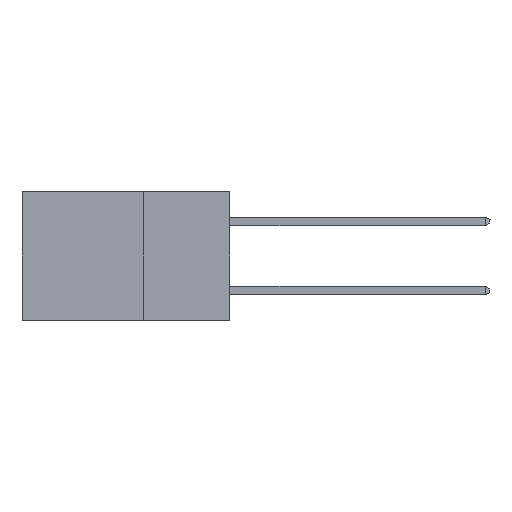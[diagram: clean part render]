
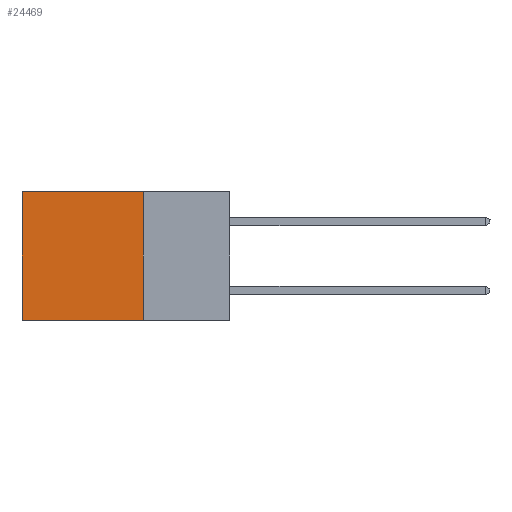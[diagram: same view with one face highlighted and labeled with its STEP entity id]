
A CAD part, left-side view. The second image highlights one B-rep face of the part: STEP entity #24469.
In plain terms, the highlighted planar face has unit normal (-1, 0, 0).
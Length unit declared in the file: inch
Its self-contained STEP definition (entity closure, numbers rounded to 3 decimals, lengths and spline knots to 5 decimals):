
#397 = CARTESIAN_POINT ( 'NONE',  ( 0.298, 0.6, 0. ) ) ;
#548 = FACE_OUTER_BOUND ( 'NONE', #2076, .T. ) ;
#900 = CARTESIAN_POINT ( 'NONE',  ( 0.298, 0.6, 0. ) ) ;
#1312 = LINE ( 'NONE', #29247, #14304 ) ;
#1994 = CARTESIAN_POINT ( 'NONE',  ( 0.298, 0.25, -0.37 ) ) ;
#2076 = EDGE_LOOP ( 'NONE', ( #16856, #30841, #19656, #23746 ) ) ;
#3629 = LINE ( 'NONE', #1994, #8126 ) ;
#5730 = CARTESIAN_POINT ( 'NONE',  ( 0.298, 0.25, 0. ) ) ;
#8126 = VECTOR ( 'NONE', #17447, 39.37008 ) ;
#8401 = PLANE ( 'NONE',  #29562 ) ;
#10236 = LINE ( 'NONE', #12676, #28833 ) ;
#11460 = VERTEX_POINT ( 'NONE', #15245 ) ;
#12676 = CARTESIAN_POINT ( 'NONE',  ( 0.298, 0.25, 0. ) ) ;
#12886 = CARTESIAN_POINT ( 'NONE',  ( 0.298, 0.6, -0.37 ) ) ;
#13805 = EDGE_CURVE ( 'NONE', #15406, #20368, #27238, .T. ) ;
#13958 = DIRECTION ( 'NONE',  ( 0., 0., -1. ) ) ;
#14078 = DIRECTION ( 'NONE',  ( 1., 0., 0. ) ) ;
#14304 = VECTOR ( 'NONE', #31786, 39.37008 ) ;
#15245 = CARTESIAN_POINT ( 'NONE',  ( 0.298, 0.25, -0.37 ) ) ;
#15264 = EDGE_CURVE ( 'NONE', #11460, #20368, #3629, .T. ) ;
#15386 = DIRECTION ( 'NONE',  ( 0., 1., 0. ) ) ;
#15406 = VERTEX_POINT ( 'NONE', #397 ) ;
#16856 = ORIENTED_EDGE ( 'NONE', *, *, #13805, .T. ) ;
#17447 = DIRECTION ( 'NONE',  ( 0., 1., 0. ) ) ;
#19385 = EDGE_CURVE ( 'NONE', #26998, #11460, #1312, .T. ) ;
#19656 = ORIENTED_EDGE ( 'NONE', *, *, #19385, .F. ) ;
#20368 = VERTEX_POINT ( 'NONE', #12886 ) ;
#20542 = VECTOR ( 'NONE', #13958, 39.37008 ) ;
#23746 = ORIENTED_EDGE ( 'NONE', *, *, #25484, .T. ) ;
#24469 = ADVANCED_FACE ( 'NONE', ( #548 ), #8401, .F. ) ;
#25484 = EDGE_CURVE ( 'NONE', #26998, #15406, #10236, .T. ) ;
#26998 = VERTEX_POINT ( 'NONE', #5730 ) ;
#27238 = LINE ( 'NONE', #900, #20542 ) ;
#28833 = VECTOR ( 'NONE', #15386, 39.37008 ) ;
#29147 = CARTESIAN_POINT ( 'NONE',  ( 0.298, 0.25, 0. ) ) ;
#29247 = CARTESIAN_POINT ( 'NONE',  ( 0.298, 0.25, 0. ) ) ;
#29562 = AXIS2_PLACEMENT_3D ( 'NONE', #29147, #14078, #31684 ) ;
#30841 = ORIENTED_EDGE ( 'NONE', *, *, #15264, .F. ) ;
#31684 = DIRECTION ( 'NONE',  ( 0., 0., -1. ) ) ;
#31786 = DIRECTION ( 'NONE',  ( 0., 0., -1. ) ) ;
